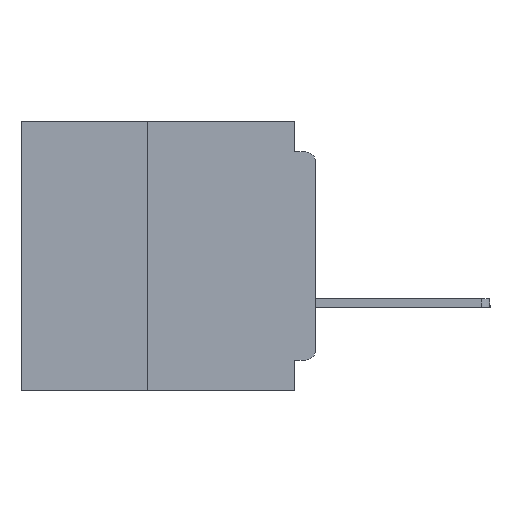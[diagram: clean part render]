
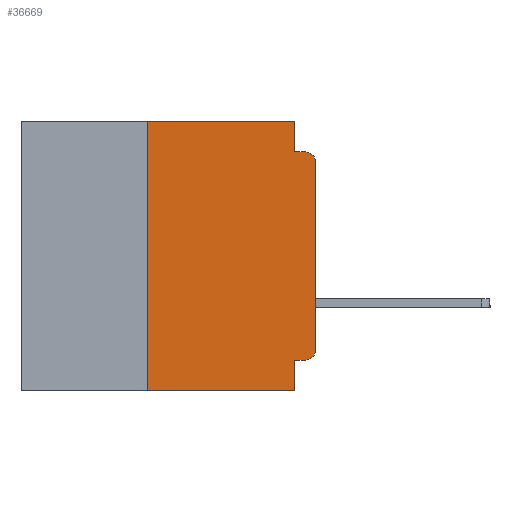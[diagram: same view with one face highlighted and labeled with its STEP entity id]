
A CAD part, left-side view. The second image highlights one B-rep face of the part: STEP entity #36669.
In plain terms, the highlighted planar face has unit normal (-1, 0, 0).
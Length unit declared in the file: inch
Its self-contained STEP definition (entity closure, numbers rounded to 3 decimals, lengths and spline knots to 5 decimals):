
#447 = VECTOR ( 'NONE', #59309, 39.37008 ) ;
#1581 = DIRECTION ( 'NONE',  ( 1., 0., 0. ) ) ;
#2026 = LINE ( 'NONE', #54398, #447 ) ;
#2260 = EDGE_CURVE ( 'NONE', #54448, #44606, #45816, .T. ) ;
#2572 = EDGE_CURVE ( 'NONE', #5341, #12603, #40327, .T. ) ;
#4533 = ORIENTED_EDGE ( 'NONE', *, *, #2260, .T. ) ;
#5341 = VERTEX_POINT ( 'NONE', #47079 ) ;
#6834 = FACE_OUTER_BOUND ( 'NONE', #38271, .T. ) ;
#8665 = VECTOR ( 'NONE', #12346, 39.37008 ) ;
#8711 = CARTESIAN_POINT ( 'NONE',  ( 0., 0., -0.355 ) ) ;
#9477 = CIRCLE ( 'NONE', #11484, 0.015 ) ;
#9738 = VERTEX_POINT ( 'NONE', #53170 ) ;
#10399 = VERTEX_POINT ( 'NONE', #28272 ) ;
#11484 = AXIS2_PLACEMENT_3D ( 'NONE', #23037, #57806, #28072 ) ;
#12069 = CARTESIAN_POINT ( 'NONE',  ( 0., 0.031, 0. ) ) ;
#12346 = DIRECTION ( 'NONE',  ( 0., -1., 0. ) ) ;
#12603 = VERTEX_POINT ( 'NONE', #12069 ) ;
#12645 = DIRECTION ( 'NONE',  ( 0., 0., -1. ) ) ;
#12725 = DIRECTION ( 'NONE',  ( -1., 0., 0. ) ) ;
#13156 = CARTESIAN_POINT ( 'NONE',  ( 0., 0.015, -0.34 ) ) ;
#16193 = CARTESIAN_POINT ( 'NONE',  ( 0., 0.031, 0. ) ) ;
#17382 = EDGE_CURVE ( 'NONE', #9738, #5341, #21127, .T. ) ;
#18526 = CARTESIAN_POINT ( 'NONE',  ( 0., 0., -0.06 ) ) ;
#18689 = VECTOR ( 'NONE', #43621, 39.37008 ) ;
#19285 = ORIENTED_EDGE ( 'NONE', *, *, #46389, .F. ) ;
#19471 = LINE ( 'NONE', #16193, #31195 ) ;
#20314 = ORIENTED_EDGE ( 'NONE', *, *, #29148, .F. ) ;
#21127 = LINE ( 'NONE', #41090, #34436 ) ;
#21481 = AXIS2_PLACEMENT_3D ( 'NONE', #13156, #12725, #12645 ) ;
#21726 = VECTOR ( 'NONE', #52237, 39.37008 ) ;
#21898 = LINE ( 'NONE', #46973, #8665 ) ;
#22522 = ORIENTED_EDGE ( 'NONE', *, *, #37688, .T. ) ;
#23037 = CARTESIAN_POINT ( 'NONE',  ( 0., 0.015, -0.06 ) ) ;
#23432 = CARTESIAN_POINT ( 'NONE',  ( 0., 0.031, -0.4 ) ) ;
#23762 = EDGE_CURVE ( 'NONE', #33165, #10399, #9477, .T. ) ;
#26991 = VECTOR ( 'NONE', #58946, 39.37008 ) ;
#28072 = DIRECTION ( 'NONE',  ( 0., 0., -1. ) ) ;
#28272 = CARTESIAN_POINT ( 'NONE',  ( 0., 0.015, -0.045 ) ) ;
#29148 = EDGE_CURVE ( 'NONE', #54448, #55289, #46718, .T. ) ;
#29542 = CARTESIAN_POINT ( 'NONE',  ( 0., 0.015, -0.355 ) ) ;
#31051 = DIRECTION ( 'NONE',  ( 0., 0., 1. ) ) ;
#31195 = VECTOR ( 'NONE', #50987, 39.37008 ) ;
#31493 = CARTESIAN_POINT ( 'NONE',  ( 0., 0.437, 0. ) ) ;
#31958 = DIRECTION ( 'NONE',  ( 0., 0., 1. ) ) ;
#32520 = ORIENTED_EDGE ( 'NONE', *, *, #17382, .F. ) ;
#33165 = VERTEX_POINT ( 'NONE', #18526 ) ;
#33314 = LINE ( 'NONE', #61643, #49118 ) ;
#34436 = VECTOR ( 'NONE', #31051, 39.37008 ) ;
#36510 = DIRECTION ( 'NONE',  ( 0., 0., -1. ) ) ;
#36593 = LINE ( 'NONE', #37312, #21726 ) ;
#36669 = ADVANCED_FACE ( 'NONE', ( #6834 ), #56224, .F. ) ;
#37312 = CARTESIAN_POINT ( 'NONE',  ( 0., 0.031, -0.4 ) ) ;
#37688 = EDGE_CURVE ( 'NONE', #9738, #49492, #2026, .T. ) ;
#38271 = EDGE_LOOP ( 'NONE', ( #62040, #62820, #60475, #19285, #42724, #32520, #22522, #39105, #20314, #4533 ) ) ;
#39105 = ORIENTED_EDGE ( 'NONE', *, *, #46947, .F. ) ;
#40327 = LINE ( 'NONE', #59455, #26991 ) ;
#41090 = CARTESIAN_POINT ( 'NONE',  ( 0., 0.25, -0.4 ) ) ;
#42651 = EDGE_CURVE ( 'NONE', #49458, #10399, #21898, .T. ) ;
#42724 = ORIENTED_EDGE ( 'NONE', *, *, #2572, .F. ) ;
#43621 = DIRECTION ( 'NONE',  ( 0., 1., 0. ) ) ;
#44606 = VERTEX_POINT ( 'NONE', #56201 ) ;
#44712 = CARTESIAN_POINT ( 'NONE',  ( 0., 0.031, -0.355 ) ) ;
#45816 = CIRCLE ( 'NONE', #21481, 0.015 ) ;
#45914 = EDGE_CURVE ( 'NONE', #44606, #33165, #33314, .T. ) ;
#46389 = EDGE_CURVE ( 'NONE', #12603, #49458, #19471, .T. ) ;
#46718 = LINE ( 'NONE', #8711, #18689 ) ;
#46947 = EDGE_CURVE ( 'NONE', #55289, #49492, #36593, .T. ) ;
#46973 = CARTESIAN_POINT ( 'NONE',  ( 0., 0., -0.045 ) ) ;
#47079 = CARTESIAN_POINT ( 'NONE',  ( 0., 0.25, 0. ) ) ;
#49118 = VECTOR ( 'NONE', #31958, 39.37008 ) ;
#49458 = VERTEX_POINT ( 'NONE', #53050 ) ;
#49492 = VERTEX_POINT ( 'NONE', #23432 ) ;
#50987 = DIRECTION ( 'NONE',  ( 0., 0., -1. ) ) ;
#52237 = DIRECTION ( 'NONE',  ( 0., 0., -1. ) ) ;
#53050 = CARTESIAN_POINT ( 'NONE',  ( 0., 0.031, -0.045 ) ) ;
#53170 = CARTESIAN_POINT ( 'NONE',  ( 0., 0.25, -0.4 ) ) ;
#54398 = CARTESIAN_POINT ( 'NONE',  ( 0., 0.437, -0.4 ) ) ;
#54448 = VERTEX_POINT ( 'NONE', #29542 ) ;
#55289 = VERTEX_POINT ( 'NONE', #44712 ) ;
#56201 = CARTESIAN_POINT ( 'NONE',  ( 0., 0., -0.34 ) ) ;
#56224 = PLANE ( 'NONE',  #61401 ) ;
#57806 = DIRECTION ( 'NONE',  ( -1., 0., 0. ) ) ;
#58946 = DIRECTION ( 'NONE',  ( 0., -1., 0. ) ) ;
#59309 = DIRECTION ( 'NONE',  ( 0., -1., 0. ) ) ;
#59455 = CARTESIAN_POINT ( 'NONE',  ( 0., 0.437, 0. ) ) ;
#60475 = ORIENTED_EDGE ( 'NONE', *, *, #42651, .F. ) ;
#61401 = AXIS2_PLACEMENT_3D ( 'NONE', #31493, #1581, #36510 ) ;
#61643 = CARTESIAN_POINT ( 'NONE',  ( 0., 0., 0. ) ) ;
#62040 = ORIENTED_EDGE ( 'NONE', *, *, #45914, .T. ) ;
#62820 = ORIENTED_EDGE ( 'NONE', *, *, #23762, .T. ) ;
